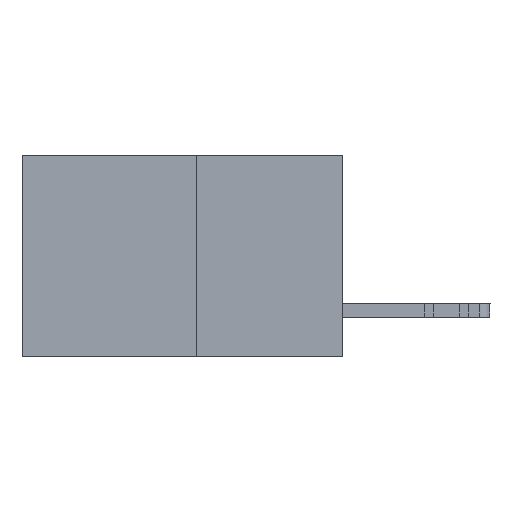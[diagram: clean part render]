
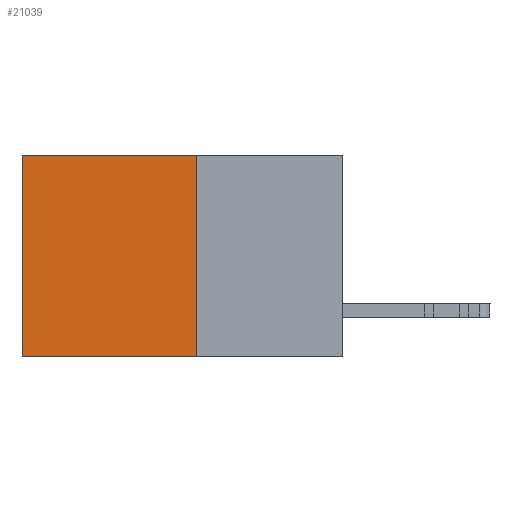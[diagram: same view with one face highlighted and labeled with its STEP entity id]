
A CAD part, left-side view. The second image highlights one B-rep face of the part: STEP entity #21039.
In plain terms, the highlighted planar face has unit normal (-1, 0, 0).
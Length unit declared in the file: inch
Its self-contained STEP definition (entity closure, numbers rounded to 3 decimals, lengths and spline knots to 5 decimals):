
#140 = VECTOR ( 'NONE', #24226, 39.37008 ) ;
#326 = LINE ( 'NONE', #8807, #21702 ) ;
#1346 = ORIENTED_EDGE ( 'NONE', *, *, #3602, .F. ) ;
#2715 = LINE ( 'NONE', #11069, #3542 ) ;
#3542 = VECTOR ( 'NONE', #13633, 39.37008 ) ;
#3602 = EDGE_CURVE ( 'NONE', #24480, #20943, #18885, .T. ) ;
#4600 = DIRECTION ( 'NONE',  ( 1., 0., 0. ) ) ;
#5396 = CARTESIAN_POINT ( 'NONE',  ( 0.277, 0.27, -0.37 ) ) ;
#6047 = ORIENTED_EDGE ( 'NONE', *, *, #11920, .T. ) ;
#6537 = FACE_OUTER_BOUND ( 'NONE', #12539, .T. ) ;
#7110 = LINE ( 'NONE', #24109, #140 ) ;
#8521 = VERTEX_POINT ( 'NONE', #29534 ) ;
#8807 = CARTESIAN_POINT ( 'NONE',  ( 0.277, 0.59, -0.37 ) ) ;
#9561 = ORIENTED_EDGE ( 'NONE', *, *, #25878, .T. ) ;
#11069 = CARTESIAN_POINT ( 'NONE',  ( 0.277, 0.27, 0. ) ) ;
#11215 = DIRECTION ( 'NONE',  ( 0., 1., 0. ) ) ;
#11920 = EDGE_CURVE ( 'NONE', #8521, #20943, #326, .T. ) ;
#12267 = CARTESIAN_POINT ( 'NONE',  ( 0.277, 0.27, -0.37 ) ) ;
#12539 = EDGE_LOOP ( 'NONE', ( #6047, #1346, #20737, #9561 ) ) ;
#13633 = DIRECTION ( 'NONE',  ( 0., 1., 0. ) ) ;
#16051 = CARTESIAN_POINT ( 'NONE',  ( 0.277, 0.27, 0. ) ) ;
#17635 = VERTEX_POINT ( 'NONE', #16051 ) ;
#17779 = EDGE_CURVE ( 'NONE', #17635, #24480, #7110, .T. ) ;
#18073 = VECTOR ( 'NONE', #11215, 39.37008 ) ;
#18885 = LINE ( 'NONE', #24064, #18073 ) ;
#19944 = PLANE ( 'NONE',  #26313 ) ;
#20737 = ORIENTED_EDGE ( 'NONE', *, *, #17779, .F. ) ;
#20943 = VERTEX_POINT ( 'NONE', #32552 ) ;
#21039 = ADVANCED_FACE ( 'NONE', ( #6537 ), #19944, .F. ) ;
#21702 = VECTOR ( 'NONE', #29293, 39.37008 ) ;
#22522 = DIRECTION ( 'NONE',  ( 0., 0., -1. ) ) ;
#24064 = CARTESIAN_POINT ( 'NONE',  ( 0.277, 0.27, -0.37 ) ) ;
#24109 = CARTESIAN_POINT ( 'NONE',  ( 0.277, 0.27, -0.37 ) ) ;
#24226 = DIRECTION ( 'NONE',  ( 0., 0., -1. ) ) ;
#24480 = VERTEX_POINT ( 'NONE', #5396 ) ;
#25878 = EDGE_CURVE ( 'NONE', #17635, #8521, #2715, .T. ) ;
#26313 = AXIS2_PLACEMENT_3D ( 'NONE', #12267, #4600, #22522 ) ;
#29293 = DIRECTION ( 'NONE',  ( 0., 0., -1. ) ) ;
#29534 = CARTESIAN_POINT ( 'NONE',  ( 0.277, 0.59, 0. ) ) ;
#32552 = CARTESIAN_POINT ( 'NONE',  ( 0.277, 0.59, -0.37 ) ) ;
